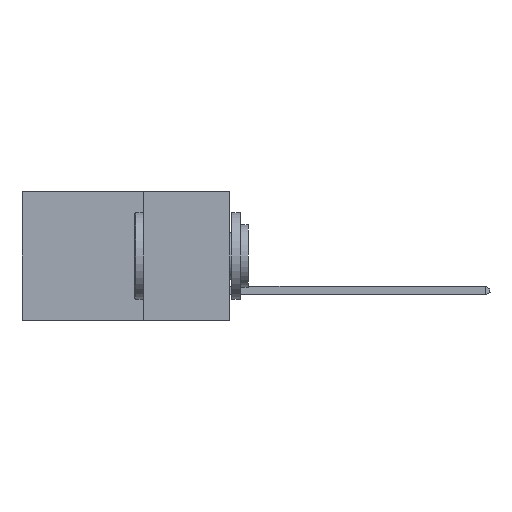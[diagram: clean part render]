
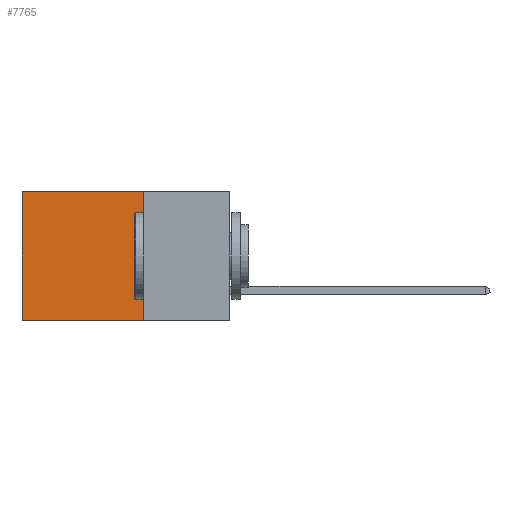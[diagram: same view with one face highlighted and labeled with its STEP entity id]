
A CAD part, left-side view. The second image highlights one B-rep face of the part: STEP entity #7765.
In plain terms, the highlighted planar face has unit normal (-1, 0, 0).
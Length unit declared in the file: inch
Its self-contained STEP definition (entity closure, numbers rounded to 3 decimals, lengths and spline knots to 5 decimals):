
#221 = CARTESIAN_POINT ( 'NONE',  ( 0.298, 0.25, -0.37 ) ) ;
#636 = EDGE_CURVE ( 'NONE', #11214, #6098, #8758, .T. ) ;
#1457 = LINE ( 'NONE', #5241, #18641 ) ;
#1460 = LINE ( 'NONE', #11340, #17859 ) ;
#2141 = PLANE ( 'NONE',  #7312 ) ;
#4006 = VECTOR ( 'NONE', #8546, 39.37008 ) ;
#4210 = VECTOR ( 'NONE', #7555, 39.37008 ) ;
#5241 = CARTESIAN_POINT ( 'NONE',  ( 0.298, 0.25, 0. ) ) ;
#5402 = CARTESIAN_POINT ( 'NONE',  ( 0.298, 0.25, 0. ) ) ;
#6098 = VERTEX_POINT ( 'NONE', #11730 ) ;
#6854 = DIRECTION ( 'NONE',  ( 0., 1., 0. ) ) ;
#6899 = ORIENTED_EDGE ( 'NONE', *, *, #18699, .F. ) ;
#7312 = AXIS2_PLACEMENT_3D ( 'NONE', #18706, #20394, #11970 ) ;
#7555 = DIRECTION ( 'NONE',  ( 0., 1., 0. ) ) ;
#7558 = EDGE_LOOP ( 'NONE', ( #9976, #11010, #6899, #13436 ) ) ;
#7765 = ADVANCED_FACE ( 'NONE', ( #10187 ), #2141, .F. ) ;
#8546 = DIRECTION ( 'NONE',  ( 0., 0., -1. ) ) ;
#8758 = LINE ( 'NONE', #11686, #4006 ) ;
#9976 = ORIENTED_EDGE ( 'NONE', *, *, #636, .T. ) ;
#10187 = FACE_OUTER_BOUND ( 'NONE', #7558, .T. ) ;
#10938 = EDGE_CURVE ( 'NONE', #11857, #6098, #15032, .T. ) ;
#11010 = ORIENTED_EDGE ( 'NONE', *, *, #10938, .F. ) ;
#11214 = VERTEX_POINT ( 'NONE', #20868 ) ;
#11340 = CARTESIAN_POINT ( 'NONE',  ( 0.298, 0.25, 0. ) ) ;
#11686 = CARTESIAN_POINT ( 'NONE',  ( 0.298, 0.6, 0. ) ) ;
#11730 = CARTESIAN_POINT ( 'NONE',  ( 0.298, 0.6, -0.37 ) ) ;
#11857 = VERTEX_POINT ( 'NONE', #221 ) ;
#11970 = DIRECTION ( 'NONE',  ( 0., 0., -1. ) ) ;
#13436 = ORIENTED_EDGE ( 'NONE', *, *, #19906, .T. ) ;
#15032 = LINE ( 'NONE', #21303, #4210 ) ;
#16075 = VERTEX_POINT ( 'NONE', #5402 ) ;
#17859 = VECTOR ( 'NONE', #18132, 39.37008 ) ;
#18132 = DIRECTION ( 'NONE',  ( 0., 0., -1. ) ) ;
#18641 = VECTOR ( 'NONE', #6854, 39.37008 ) ;
#18699 = EDGE_CURVE ( 'NONE', #16075, #11857, #1460, .T. ) ;
#18706 = CARTESIAN_POINT ( 'NONE',  ( 0.298, 0.25, 0. ) ) ;
#19906 = EDGE_CURVE ( 'NONE', #16075, #11214, #1457, .T. ) ;
#20394 = DIRECTION ( 'NONE',  ( 1., 0., 0. ) ) ;
#20868 = CARTESIAN_POINT ( 'NONE',  ( 0.298, 0.6, 0. ) ) ;
#21303 = CARTESIAN_POINT ( 'NONE',  ( 0.298, 0.25, -0.37 ) ) ;
